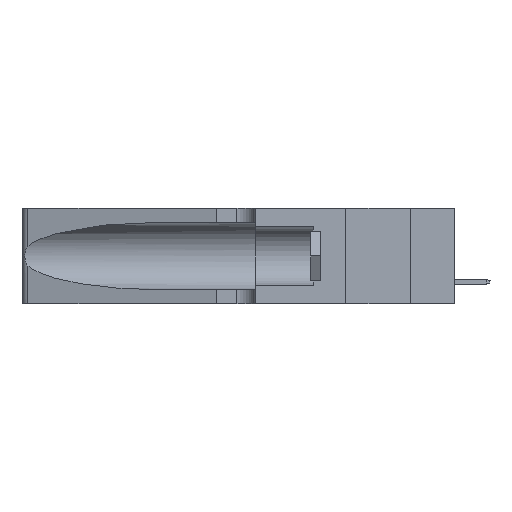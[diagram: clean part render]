
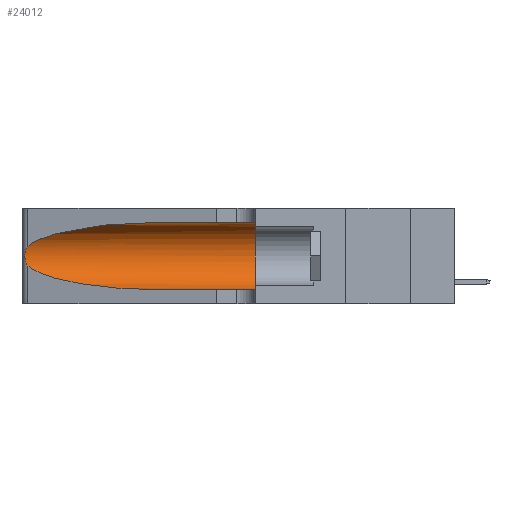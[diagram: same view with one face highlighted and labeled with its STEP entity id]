
A CAD part, left-side view. The second image highlights one B-rep face of the part: STEP entity #24012.
In plain terms, the highlighted cylindrical face has radius 3.308 mm (diameter 6.617 mm), a partial arc.
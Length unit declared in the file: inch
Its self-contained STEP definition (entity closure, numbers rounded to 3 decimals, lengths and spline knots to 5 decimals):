
#40 = DIRECTION ( 'NONE',  ( 0., 0., -1. ) ) ;
#223 = CARTESIAN_POINT ( 'NONE',  ( 0.25555, 1.22993, 0.14849 ) ) ;
#2424 = EDGE_CURVE ( 'NONE', #2530, #8594, #18812, .T. ) ;
#2530 = VERTEX_POINT ( 'NONE', #37899 ) ;
#3919 = ORIENTED_EDGE ( 'NONE', *, *, #15680, .F. ) ;
#4595 = LINE ( 'NONE', #41423, #14725 ) ;
#5542 = CIRCLE ( 'NONE', #8586, 0.13025 ) ;
#6804 = CARTESIAN_POINT ( 'NONE',  ( 0.1305, 0.35, 0.185 ) ) ;
#7525 = CARTESIAN_POINT ( 'NONE',  ( 0.1305, 1.61858, 0.05475 ) ) ;
#7568 = CARTESIAN_POINT ( 'NONE',  ( 0.2373, 1.15595, 0.08982 ) ) ;
#7644 = CARTESIAN_POINT ( 'NONE',  ( 0.25487, 1.22718, 0.22369 ) ) ;
#8152 = CARTESIAN_POINT ( 'NONE',  ( 0.25487, 1.22718, 0.14631 ) ) ;
#8586 = AXIS2_PLACEMENT_3D ( 'NONE', #6804, #43629, #14041 ) ;
#8594 = VERTEX_POINT ( 'NONE', #13703 ) ;
#8728 = EDGE_CURVE ( 'NONE', #25408, #16504, #40704, .T. ) ;
#9803 = DIRECTION ( 'NONE',  ( 0., -1., 0. ) ) ;
#10410 = CARTESIAN_POINT ( 'NONE',  ( 0.1305, 1.61858, 0.185 ) ) ;
#11276 = CARTESIAN_POINT ( 'NONE',  ( 0.26075, 1.23896, 0.19203 ) ) ;
#11992 = ORIENTED_EDGE ( 'NONE', *, *, #8728, .T. ) ;
#13703 = CARTESIAN_POINT ( 'NONE',  ( 0.1305, 0.35, 0.05475 ) ) ;
#13826 = ORIENTED_EDGE ( 'NONE', *, *, #27704, .T. ) ;
#14041 = DIRECTION ( 'NONE',  ( 0., 0., 1. ) ) ;
#14725 = VECTOR ( 'NONE', #9803, 39.37008 ) ;
#15121 = CARTESIAN_POINT ( 'NONE',  ( 0.25555, 1.22994, 0.2215 ) ) ;
#15168 = VECTOR ( 'NONE', #43641, 39.37008 ) ;
#15172 = CARTESIAN_POINT ( 'NONE',  ( 0.25487, 1.22718, 0.14631 ) ) ;
#15680 = EDGE_CURVE ( 'NONE', #16575, #8594, #5542, .T. ) ;
#16504 = VERTEX_POINT ( 'NONE', #15172 ) ;
#16551 = AXIS2_PLACEMENT_3D ( 'NONE', #10410, #25791, #40 ) ;
#16575 = VERTEX_POINT ( 'NONE', #32782 ) ;
#18369 =( BOUNDED_CURVE ( )  B_SPLINE_CURVE ( 3, ( #18452, #44246, #22318, #7644 ),
 .UNSPECIFIED., .F., .F. ) 
 B_SPLINE_CURVE_WITH_KNOTS ( ( 4, 4 ),
 ( 1.5708, 2.84003 ),
 .UNSPECIFIED. ) 
 CURVE ( )  GEOMETRIC_REPRESENTATION_ITEM ( )  RATIONAL_B_SPLINE_CURVE ( ( 1., 0.87, 0.87, 1. ) ) 
 REPRESENTATION_ITEM ( '' )  );
#18452 = CARTESIAN_POINT ( 'NONE',  ( 0.1305, 0.72297, 0.31525 ) ) ;
#18620 = CARTESIAN_POINT ( 'NONE',  ( 0.25487, 1.22718, 0.14631 ) ) ;
#18812 = LINE ( 'NONE', #7525, #15168 ) ;
#18941 = CARTESIAN_POINT ( 'NONE',  ( 0.26017, 1.23833, 0.17102 ) ) ;
#19265 = ORIENTED_EDGE ( 'NONE', *, *, #44045, .F. ) ;
#22318 = CARTESIAN_POINT ( 'NONE',  ( 0.2373, 1.15595, 0.28018 ) ) ;
#22332 = CARTESIAN_POINT ( 'NONE',  ( 0.26075, 1.23896, 0.178 ) ) ;
#22583 = CARTESIAN_POINT ( 'NONE',  ( 0.25639, 1.23186, 0.15144 ) ) ;
#24012 = ADVANCED_FACE ( 'NONE', ( #47235 ), #33041, .F. ) ;
#25408 = VERTEX_POINT ( 'NONE', #47016 ) ;
#25791 = DIRECTION ( 'NONE',  ( 0., -1., 0. ) ) ;
#25959 = CARTESIAN_POINT ( 'NONE',  ( 0.25789, 1.23486, 0.15765 ) ) ;
#27704 = EDGE_CURVE ( 'NONE', #46895, #25408, #18369, .T. ) ;
#29326 = CARTESIAN_POINT ( 'NONE',  ( 0.25856, 1.23593, 0.16098 ) ) ;
#29806 = CARTESIAN_POINT ( 'NONE',  ( 0.25487, 1.22718, 0.22369 ) ) ;
#32782 = CARTESIAN_POINT ( 'NONE',  ( 0.1305, 0.35, 0.31525 ) ) ;
#32884 = CARTESIAN_POINT ( 'NONE',  ( 0.1305, 0.72297, 0.05475 ) ) ;
#32972 = CARTESIAN_POINT ( 'NONE',  ( 0.25787, 1.23484, 0.2124 ) ) ;
#33041 = CYLINDRICAL_SURFACE ( 'NONE', #16551, 0.13025 ) ;
#36152 = EDGE_LOOP ( 'NONE', ( #13826, #11992, #40335, #43896, #3919, #19265 ) ) ;
#36502 = CARTESIAN_POINT ( 'NONE',  ( 0.1305, 0.72297, 0.31525 ) ) ;
#36979 = CARTESIAN_POINT ( 'NONE',  ( 0.18966, 0.96281, 0.05475 ) ) ;
#37899 = CARTESIAN_POINT ( 'NONE',  ( 0.1305, 0.72297, 0.05475 ) ) ;
#40335 = ORIENTED_EDGE ( 'NONE', *, *, #41829, .T. ) ;
#40704 = B_SPLINE_CURVE_WITH_KNOTS ( 'NONE', 3,
 ( #29806, #15121, #44730, #32972, #41140, #44487, #11276, #22332, #18941, #29326, #25959, #22583, #223, #8152 ),
 .UNSPECIFIED., .F., .F.,
 ( 4, 2, 2, 2, 2, 2, 4 ),
 ( 0., 0.00027, 0.00053, 0.00107, 0.0016, 0.00187, 0.00214 ),
 .UNSPECIFIED. ) ;
#40919 =( BOUNDED_CURVE ( )  B_SPLINE_CURVE ( 3, ( #18620, #7568, #36979, #32884 ),
 .UNSPECIFIED., .F., .F. ) 
 B_SPLINE_CURVE_WITH_KNOTS ( ( 4, 4 ),
 ( 3.44316, 4.71239 ),
 .UNSPECIFIED. ) 
 CURVE ( )  GEOMETRIC_REPRESENTATION_ITEM ( )  RATIONAL_B_SPLINE_CURVE ( ( 1., 0.87, 0.87, 1. ) ) 
 REPRESENTATION_ITEM ( '' )  );
#41140 = CARTESIAN_POINT ( 'NONE',  ( 0.25854, 1.2359, 0.20912 ) ) ;
#41423 = CARTESIAN_POINT ( 'NONE',  ( 0.1305, 1.61858, 0.31525 ) ) ;
#41829 = EDGE_CURVE ( 'NONE', #16504, #2530, #40919, .T. ) ;
#43629 = DIRECTION ( 'NONE',  ( 0., 1., 0. ) ) ;
#43641 = DIRECTION ( 'NONE',  ( 0., -1., 0. ) ) ;
#43896 = ORIENTED_EDGE ( 'NONE', *, *, #2424, .T. ) ;
#44045 = EDGE_CURVE ( 'NONE', #46895, #16575, #4595, .T. ) ;
#44246 = CARTESIAN_POINT ( 'NONE',  ( 0.18966, 0.96281, 0.31525 ) ) ;
#44487 = CARTESIAN_POINT ( 'NONE',  ( 0.26018, 1.23835, 0.19895 ) ) ;
#44730 = CARTESIAN_POINT ( 'NONE',  ( 0.25639, 1.23184, 0.21858 ) ) ;
#46895 = VERTEX_POINT ( 'NONE', #36502 ) ;
#47016 = CARTESIAN_POINT ( 'NONE',  ( 0.25487, 1.22718, 0.22369 ) ) ;
#47235 = FACE_OUTER_BOUND ( 'NONE', #36152, .T. ) ;
